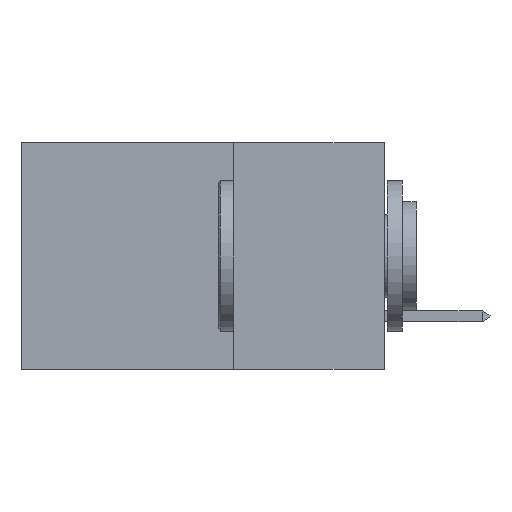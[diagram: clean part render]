
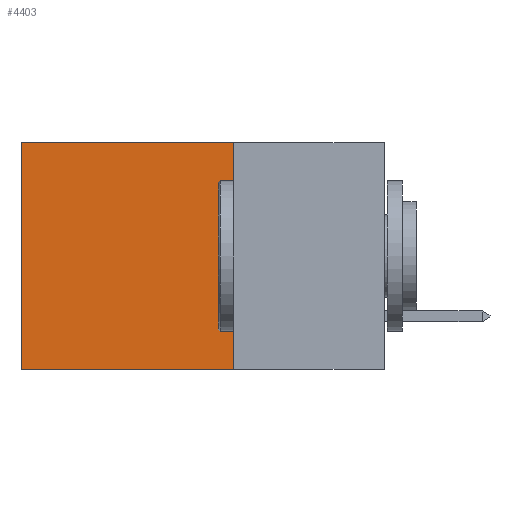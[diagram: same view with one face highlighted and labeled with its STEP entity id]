
A CAD part, left-side view. The second image highlights one B-rep face of the part: STEP entity #4403.
In plain terms, the highlighted planar face has unit normal (-1, 0, 0).
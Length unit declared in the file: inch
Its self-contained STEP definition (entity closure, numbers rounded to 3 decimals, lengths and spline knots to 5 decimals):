
#82 = VERTEX_POINT ( 'NONE', #6170 ) ;
#679 = DIRECTION ( 'NONE',  ( 0., 0., -1. ) ) ;
#965 = DIRECTION ( 'NONE',  ( 0., 0., -1. ) ) ;
#1119 = CARTESIAN_POINT ( 'NONE',  ( 0.2875, 0.6, -0.375 ) ) ;
#1280 = EDGE_CURVE ( 'NONE', #82, #3687, #4362, .T. ) ;
#1353 = AXIS2_PLACEMENT_3D ( 'NONE', #6942, #6322, #679 ) ;
#1957 = FACE_OUTER_BOUND ( 'NONE', #6973, .T. ) ;
#2104 = LINE ( 'NONE', #5815, #9032 ) ;
#2151 = CARTESIAN_POINT ( 'NONE',  ( 0.2875, 0.25, 0. ) ) ;
#2484 = VECTOR ( 'NONE', #8563, 39.37008 ) ;
#2727 = VERTEX_POINT ( 'NONE', #9058 ) ;
#3151 = ORIENTED_EDGE ( 'NONE', *, *, #1280, .F. ) ;
#3152 = ORIENTED_EDGE ( 'NONE', *, *, #8310, .T. ) ;
#3650 = DIRECTION ( 'NONE',  ( 0., 0., -1. ) ) ;
#3687 = VERTEX_POINT ( 'NONE', #1119 ) ;
#4158 = VECTOR ( 'NONE', #6870, 39.37008 ) ;
#4248 = EDGE_CURVE ( 'NONE', #7130, #82, #8777, .T. ) ;
#4362 = LINE ( 'NONE', #5162, #2484 ) ;
#4403 = ADVANCED_FACE ( 'NONE', ( #1957 ), #6829, .F. ) ;
#4614 = CARTESIAN_POINT ( 'NONE',  ( 0.2875, 0.25, -0.375 ) ) ;
#5070 = EDGE_CURVE ( 'NONE', #7130, #2727, #5150, .T. ) ;
#5150 = LINE ( 'NONE', #8941, #4158 ) ;
#5162 = CARTESIAN_POINT ( 'NONE',  ( 0.2875, 0.25, -0.375 ) ) ;
#5815 = CARTESIAN_POINT ( 'NONE',  ( 0.2875, 0.6, -0.375 ) ) ;
#6170 = CARTESIAN_POINT ( 'NONE',  ( 0.2875, 0.25, -0.375 ) ) ;
#6322 = DIRECTION ( 'NONE',  ( 1., 0., 0. ) ) ;
#6829 = PLANE ( 'NONE',  #1353 ) ;
#6870 = DIRECTION ( 'NONE',  ( 0., 1., 0. ) ) ;
#6933 = VECTOR ( 'NONE', #965, 39.37008 ) ;
#6942 = CARTESIAN_POINT ( 'NONE',  ( 0.2875, 0.25, -0.375 ) ) ;
#6973 = EDGE_LOOP ( 'NONE', ( #3152, #3151, #7489, #8850 ) ) ;
#7130 = VERTEX_POINT ( 'NONE', #2151 ) ;
#7489 = ORIENTED_EDGE ( 'NONE', *, *, #4248, .F. ) ;
#8310 = EDGE_CURVE ( 'NONE', #2727, #3687, #2104, .T. ) ;
#8563 = DIRECTION ( 'NONE',  ( 0., 1., 0. ) ) ;
#8777 = LINE ( 'NONE', #4614, #6933 ) ;
#8850 = ORIENTED_EDGE ( 'NONE', *, *, #5070, .T. ) ;
#8941 = CARTESIAN_POINT ( 'NONE',  ( 0.2875, 0.25, 0. ) ) ;
#9032 = VECTOR ( 'NONE', #3650, 39.37008 ) ;
#9058 = CARTESIAN_POINT ( 'NONE',  ( 0.2875, 0.6, 0. ) ) ;
